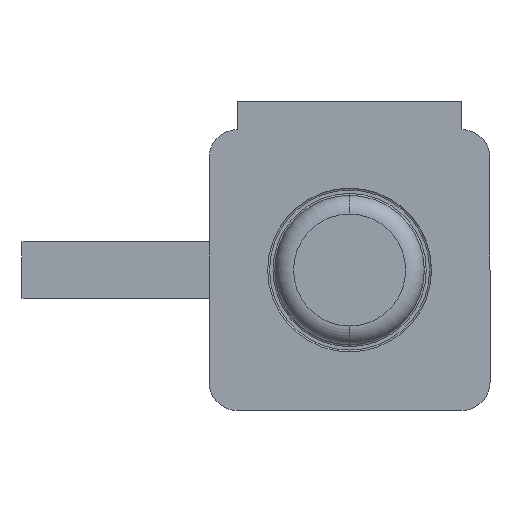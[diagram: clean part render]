
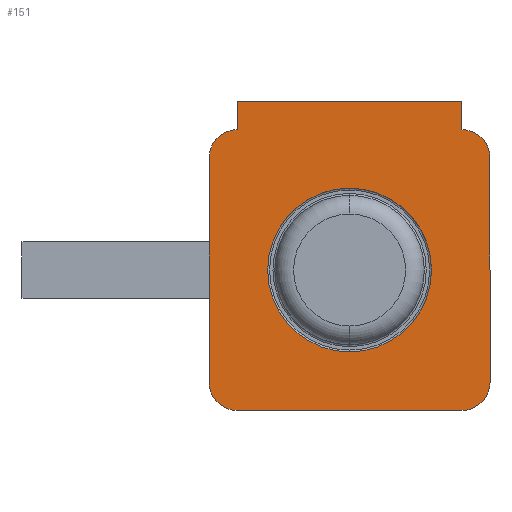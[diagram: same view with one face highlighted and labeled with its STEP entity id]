
A CAD part, front view. The second image highlights one B-rep face of the part: STEP entity #151.
In plain terms, the highlighted planar face has unit normal (0, -1, 0).
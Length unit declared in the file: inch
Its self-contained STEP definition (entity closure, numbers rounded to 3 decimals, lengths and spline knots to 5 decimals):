
#2 = AXIS2_PLACEMENT_3D ( 'NONE', #546, #30, #190 ) ;
#11 = ORIENTED_EDGE ( 'NONE', *, *, #990, .T. ) ;
#30 = DIRECTION ( 'NONE',  ( 0., -1., 0. ) ) ;
#80 = EDGE_CURVE ( 'NONE', #903, #955, #1476, .T. ) ;
#105 = CARTESIAN_POINT ( 'NONE',  ( 1.35, -2.8, 1.35 ) ) ;
#142 = ORIENTED_EDGE ( 'NONE', *, *, #373, .T. ) ;
#151 = ADVANCED_FACE ( 'NONE', ( #1006, #1975 ), #2022, .T. ) ;
#165 = DIRECTION ( 'NONE',  ( 0., 0., -1. ) ) ;
#180 = LINE ( 'NONE', #2122, #1845 ) ;
#190 = DIRECTION ( 'NONE',  ( 0., 0., -1. ) ) ;
#201 = CARTESIAN_POINT ( 'NONE',  ( 0., -2.8, 0.15 ) ) ;
#242 = CIRCLE ( 'NONE', #1972, 0.15 ) ;
#253 = EDGE_LOOP ( 'NONE', ( #1185, #807 ) ) ;
#285 = ORIENTED_EDGE ( 'NONE', *, *, #501, .T. ) ;
#294 = VERTEX_POINT ( 'NONE', #733 ) ;
#302 = DIRECTION ( 'NONE',  ( 0., -1., 0. ) ) ;
#306 = CIRCLE ( 'NONE', #308, 0.15 ) ;
#308 = AXIS2_PLACEMENT_3D ( 'NONE', #1472, #302, #1944 ) ;
#311 = DIRECTION ( 'NONE',  ( 0., 0., -1. ) ) ;
#324 = VERTEX_POINT ( 'NONE', #411 ) ;
#342 = CIRCLE ( 'NONE', #380, 0.15 ) ;
#344 = VECTOR ( 'NONE', #679, 39.37008 ) ;
#373 = EDGE_CURVE ( 'NONE', #324, #879, #242, .T. ) ;
#380 = AXIS2_PLACEMENT_3D ( 'NONE', #628, #1122, #785 ) ;
#409 = CIRCLE ( 'NONE', #2, 0.4375 ) ;
#411 = CARTESIAN_POINT ( 'NONE',  ( 1.5, -2.8, 1.35 ) ) ;
#435 = LINE ( 'NONE', #1288, #946 ) ;
#501 = EDGE_CURVE ( 'NONE', #294, #903, #342, .T. ) ;
#537 = CARTESIAN_POINT ( 'NONE',  ( 0.15, -2.8, 1.65 ) ) ;
#542 = LINE ( 'NONE', #537, #1409 ) ;
#545 = EDGE_CURVE ( 'NONE', #1035, #1112, #180, .T. ) ;
#546 = CARTESIAN_POINT ( 'NONE',  ( 0.75, -2.8, 0.75 ) ) ;
#605 = VERTEX_POINT ( 'NONE', #820 ) ;
#616 = AXIS2_PLACEMENT_3D ( 'NONE', #2003, #1001, #1859 ) ;
#628 = CARTESIAN_POINT ( 'NONE',  ( 0.15, -2.8, 1.35 ) ) ;
#679 = DIRECTION ( 'NONE',  ( 0., 0., 1. ) ) ;
#697 = LINE ( 'NONE', #880, #1529 ) ;
#716 = AXIS2_PLACEMENT_3D ( 'NONE', #1831, #1131, #1812 ) ;
#733 = CARTESIAN_POINT ( 'NONE',  ( 0.15, -2.8, 1.5 ) ) ;
#755 = ORIENTED_EDGE ( 'NONE', *, *, #545, .T. ) ;
#758 = CARTESIAN_POINT ( 'NONE',  ( 0.75, -2.8, 0.3125 ) ) ;
#785 = DIRECTION ( 'NONE',  ( 0., 0., -1. ) ) ;
#807 = ORIENTED_EDGE ( 'NONE', *, *, #1492, .F. ) ;
#820 = CARTESIAN_POINT ( 'NONE',  ( 1.5, -2.8, 0.15 ) ) ;
#821 = CARTESIAN_POINT ( 'NONE',  ( 0.15, -2.8, 0.15 ) ) ;
#843 = EDGE_CURVE ( 'NONE', #955, #1035, #1954, .T. ) ;
#879 = VERTEX_POINT ( 'NONE', #1050 ) ;
#880 = CARTESIAN_POINT ( 'NONE',  ( 0.15, -2.8, 1.65 ) ) ;
#903 = VERTEX_POINT ( 'NONE', #1202 ) ;
#946 = VECTOR ( 'NONE', #969, 39.37008 ) ;
#955 = VERTEX_POINT ( 'NONE', #201 ) ;
#969 = DIRECTION ( 'NONE',  ( 0., 0., -1. ) ) ;
#981 = DIRECTION ( 'NONE',  ( 0., -1., 0. ) ) ;
#990 = EDGE_CURVE ( 'NONE', #605, #324, #1560, .T. ) ;
#1001 = DIRECTION ( 'NONE',  ( 0., -1., 0. ) ) ;
#1006 = FACE_OUTER_BOUND ( 'NONE', #1247, .T. ) ;
#1027 = VECTOR ( 'NONE', #311, 39.37008 ) ;
#1035 = VERTEX_POINT ( 'NONE', #1541 ) ;
#1050 = CARTESIAN_POINT ( 'NONE',  ( 1.35, -2.8, 1.5 ) ) ;
#1112 = VERTEX_POINT ( 'NONE', #1843 ) ;
#1122 = DIRECTION ( 'NONE',  ( 0., -1., 0. ) ) ;
#1131 = DIRECTION ( 'NONE',  ( 0., -1., 0. ) ) ;
#1185 = ORIENTED_EDGE ( 'NONE', *, *, #2131, .F. ) ;
#1202 = CARTESIAN_POINT ( 'NONE',  ( 0., -2.8, 1.35 ) ) ;
#1212 = CARTESIAN_POINT ( 'NONE',  ( 0., -2.8, 0. ) ) ;
#1244 = DIRECTION ( 'NONE',  ( 0., -1., 0. ) ) ;
#1247 = EDGE_LOOP ( 'NONE', ( #1700, #11, #142, #1955, #1741, #1265, #285, #2109, #1374, #755 ) ) ;
#1265 = ORIENTED_EDGE ( 'NONE', *, *, #2116, .T. ) ;
#1277 = EDGE_CURVE ( 'NONE', #1552, #1343, #697, .T. ) ;
#1279 = CARTESIAN_POINT ( 'NONE',  ( 0.75, -2.8, 1.1875 ) ) ;
#1288 = CARTESIAN_POINT ( 'NONE',  ( 1.35, -2.8, 1.65 ) ) ;
#1293 = DIRECTION ( 'NONE',  ( 1., 0., 0. ) ) ;
#1325 = AXIS2_PLACEMENT_3D ( 'NONE', #821, #981, #165 ) ;
#1343 = VERTEX_POINT ( 'NONE', #1939 ) ;
#1374 = ORIENTED_EDGE ( 'NONE', *, *, #843, .T. ) ;
#1409 = VECTOR ( 'NONE', #1528, 39.37008 ) ;
#1472 = CARTESIAN_POINT ( 'NONE',  ( 1.35, -2.8, 0.15 ) ) ;
#1476 = LINE ( 'NONE', #1212, #1027 ) ;
#1492 = EDGE_CURVE ( 'NONE', #2016, #1748, #1594, .T. ) ;
#1528 = DIRECTION ( 'NONE',  ( 0., 0., -1. ) ) ;
#1529 = VECTOR ( 'NONE', #1712, 39.37008 ) ;
#1541 = CARTESIAN_POINT ( 'NONE',  ( 0.15, -2.8, 0. ) ) ;
#1552 = VERTEX_POINT ( 'NONE', #1679 ) ;
#1560 = LINE ( 'NONE', #2000, #344 ) ;
#1594 = CIRCLE ( 'NONE', #716, 0.4375 ) ;
#1679 = CARTESIAN_POINT ( 'NONE',  ( 0.15, -2.8, 1.65 ) ) ;
#1697 = EDGE_CURVE ( 'NONE', #1112, #605, #306, .T. ) ;
#1700 = ORIENTED_EDGE ( 'NONE', *, *, #1697, .T. ) ;
#1712 = DIRECTION ( 'NONE',  ( 1., 0., 0. ) ) ;
#1741 = ORIENTED_EDGE ( 'NONE', *, *, #1277, .F. ) ;
#1748 = VERTEX_POINT ( 'NONE', #1279 ) ;
#1812 = DIRECTION ( 'NONE',  ( 0., 0., -1. ) ) ;
#1831 = CARTESIAN_POINT ( 'NONE',  ( 0.75, -2.8, 0.75 ) ) ;
#1843 = CARTESIAN_POINT ( 'NONE',  ( 1.35, -2.8, 0. ) ) ;
#1845 = VECTOR ( 'NONE', #1293, 39.37008 ) ;
#1859 = DIRECTION ( 'NONE',  ( 0., 0., -1. ) ) ;
#1939 = CARTESIAN_POINT ( 'NONE',  ( 1.35, -2.8, 1.65 ) ) ;
#1944 = DIRECTION ( 'NONE',  ( 0., 0., -1. ) ) ;
#1954 = CIRCLE ( 'NONE', #1325, 0.15 ) ;
#1955 = ORIENTED_EDGE ( 'NONE', *, *, #2099, .F. ) ;
#1972 = AXIS2_PLACEMENT_3D ( 'NONE', #105, #1244, #2076 ) ;
#1975 = FACE_BOUND ( 'NONE', #253, .T. ) ;
#2000 = CARTESIAN_POINT ( 'NONE',  ( 1.5, -2.8, 0. ) ) ;
#2003 = CARTESIAN_POINT ( 'NONE',  ( 0., -2.8, 0. ) ) ;
#2016 = VERTEX_POINT ( 'NONE', #758 ) ;
#2022 = PLANE ( 'NONE',  #616 ) ;
#2076 = DIRECTION ( 'NONE',  ( 0., 0., -1. ) ) ;
#2099 = EDGE_CURVE ( 'NONE', #1343, #879, #435, .T. ) ;
#2109 = ORIENTED_EDGE ( 'NONE', *, *, #80, .T. ) ;
#2116 = EDGE_CURVE ( 'NONE', #1552, #294, #542, .T. ) ;
#2122 = CARTESIAN_POINT ( 'NONE',  ( 0., -2.8, 0. ) ) ;
#2131 = EDGE_CURVE ( 'NONE', #1748, #2016, #409, .T. ) ;
